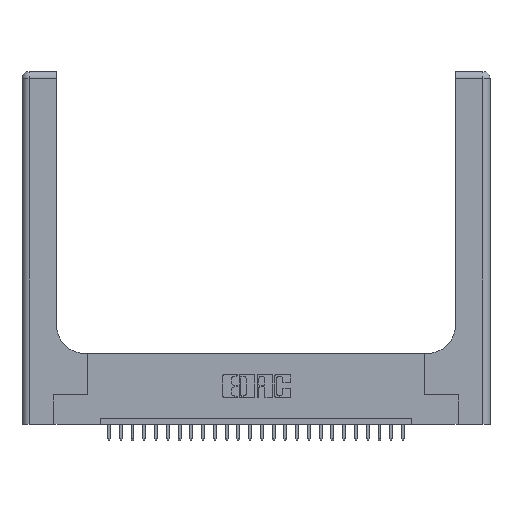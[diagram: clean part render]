
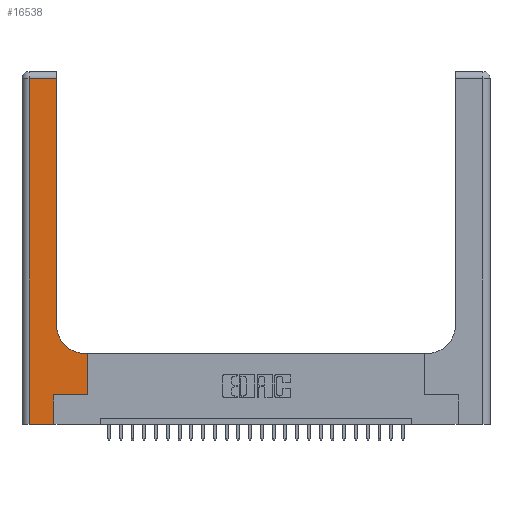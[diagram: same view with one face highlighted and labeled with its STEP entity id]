
A CAD part, top view. The second image highlights one B-rep face of the part: STEP entity #16538.
In plain terms, the highlighted planar face has unit normal (0, 0, 1).
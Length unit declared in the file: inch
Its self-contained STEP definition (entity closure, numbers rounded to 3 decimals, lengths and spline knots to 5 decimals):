
#133 = EDGE_CURVE ( 'NONE', #20920, #8429, #12386, .T. ) ;
#881 = CARTESIAN_POINT ( 'NONE',  ( 0.2915, 2.94, 0.37 ) ) ;
#912 = CARTESIAN_POINT ( 'NONE',  ( 0.269, 0.25, 0.37 ) ) ;
#1275 = CARTESIAN_POINT ( 'NONE',  ( 0.5585, 0.25, 0.37 ) ) ;
#1340 = VERTEX_POINT ( 'NONE', #8957 ) ;
#1815 = DIRECTION ( 'NONE',  ( -1., 0., 0. ) ) ;
#1842 = CARTESIAN_POINT ( 'NONE',  ( 0., 0., 0.37 ) ) ;
#2418 = CARTESIAN_POINT ( 'NONE',  ( 0.2915, 3., 0.37 ) ) ;
#2568 = AXIS2_PLACEMENT_3D ( 'NONE', #23053, #19251, #6483 ) ;
#2931 = ORIENTED_EDGE ( 'NONE', *, *, #11171, .T. ) ;
#3257 = VECTOR ( 'NONE', #15285, 39.37008 ) ;
#3536 = DIRECTION ( 'NONE',  ( 0., -1., 0. ) ) ;
#3812 = PLANE ( 'NONE',  #5685 ) ;
#4595 = CARTESIAN_POINT ( 'NONE',  ( 0.06, 3., 0.37 ) ) ;
#5685 = AXIS2_PLACEMENT_3D ( 'NONE', #11863, #24421, #1815 ) ;
#5955 = CARTESIAN_POINT ( 'NONE',  ( 0.5585, 0.25, 0.37 ) ) ;
#6483 = DIRECTION ( 'NONE',  ( 1., 0., 0. ) ) ;
#7646 = CARTESIAN_POINT ( 'NONE',  ( 0.06, 0., 0.37 ) ) ;
#7687 = EDGE_CURVE ( 'NONE', #18213, #26348, #25379, .T. ) ;
#8152 = VECTOR ( 'NONE', #20472, 39.37008 ) ;
#8415 = VERTEX_POINT ( 'NONE', #1275 ) ;
#8429 = VERTEX_POINT ( 'NONE', #22022 ) ;
#8957 = CARTESIAN_POINT ( 'NONE',  ( 0.06, 2.94, 0.37 ) ) ;
#9276 = EDGE_CURVE ( 'NONE', #23589, #14452, #10501, .T. ) ;
#9487 = LINE ( 'NONE', #1842, #12376 ) ;
#9534 = CARTESIAN_POINT ( 'NONE',  ( 0.2915, 0.85, 0.37 ) ) ;
#9589 = EDGE_CURVE ( 'NONE', #26348, #1340, #15930, .T. ) ;
#10134 = DIRECTION ( 'NONE',  ( 0., 1., 0. ) ) ;
#10501 = LINE ( 'NONE', #20712, #26354 ) ;
#11171 = EDGE_CURVE ( 'NONE', #8415, #20920, #16466, .T. ) ;
#11538 = DIRECTION ( 'NONE',  ( 1., 0., 0. ) ) ;
#11863 = CARTESIAN_POINT ( 'NONE',  ( 0., 3., 0.37 ) ) ;
#11864 = VERTEX_POINT ( 'NONE', #7646 ) ;
#12143 = VECTOR ( 'NONE', #11538, 39.37008 ) ;
#12376 = VECTOR ( 'NONE', #22918, 39.37008 ) ;
#12386 = LINE ( 'NONE', #22625, #8152 ) ;
#13251 = CARTESIAN_POINT ( 'NONE',  ( 0.5585, 0.6, 0.37 ) ) ;
#13759 = LINE ( 'NONE', #13884, #12143 ) ;
#13884 = CARTESIAN_POINT ( 'NONE',  ( 0.269, 0.25, 0.37 ) ) ;
#14039 = VECTOR ( 'NONE', #15152, 39.37008 ) ;
#14442 = ORIENTED_EDGE ( 'NONE', *, *, #133, .T. ) ;
#14452 = VERTEX_POINT ( 'NONE', #912 ) ;
#15152 = DIRECTION ( 'NONE',  ( 0., 1., 0. ) ) ;
#15285 = DIRECTION ( 'NONE',  ( -1., 0., 0. ) ) ;
#15414 = ORIENTED_EDGE ( 'NONE', *, *, #9589, .T. ) ;
#15624 = EDGE_CURVE ( 'NONE', #11864, #23589, #9487, .T. ) ;
#15787 = DIRECTION ( 'NONE',  ( 0., 1., 0. ) ) ;
#15930 = LINE ( 'NONE', #19354, #3257 ) ;
#16200 = FACE_OUTER_BOUND ( 'NONE', #22377, .T. ) ;
#16295 = VECTOR ( 'NONE', #3536, 39.37008 ) ;
#16466 = LINE ( 'NONE', #5955, #20723 ) ;
#16538 = ADVANCED_FACE ( 'NONE', ( #16200 ), #3812, .F. ) ;
#17745 = EDGE_CURVE ( 'NONE', #8429, #18213, #21360, .T. ) ;
#18213 = VERTEX_POINT ( 'NONE', #9534 ) ;
#18507 = ORIENTED_EDGE ( 'NONE', *, *, #22637, .T. ) ;
#19251 = DIRECTION ( 'NONE',  ( 0., 0., -1. ) ) ;
#19354 = CARTESIAN_POINT ( 'NONE',  ( 0., 2.94, 0.37 ) ) ;
#20167 = ORIENTED_EDGE ( 'NONE', *, *, #17745, .T. ) ;
#20472 = DIRECTION ( 'NONE',  ( -1., 0., 0. ) ) ;
#20712 = CARTESIAN_POINT ( 'NONE',  ( 0.269, 0., 0.37 ) ) ;
#20723 = VECTOR ( 'NONE', #15787, 39.37008 ) ;
#20920 = VERTEX_POINT ( 'NONE', #13251 ) ;
#21325 = CARTESIAN_POINT ( 'NONE',  ( 0.269, 0., 0.37 ) ) ;
#21360 = CIRCLE ( 'NONE', #2568, 0.25 ) ;
#21830 = LINE ( 'NONE', #4595, #16295 ) ;
#22022 = CARTESIAN_POINT ( 'NONE',  ( 0.5415, 0.6, 0.37 ) ) ;
#22159 = ORIENTED_EDGE ( 'NONE', *, *, #15624, .T. ) ;
#22222 = ORIENTED_EDGE ( 'NONE', *, *, #23088, .T. ) ;
#22377 = EDGE_LOOP ( 'NONE', ( #23172, #15414, #22222, #22159, #24361, #18507, #2931, #14442, #20167 ) ) ;
#22625 = CARTESIAN_POINT ( 'NONE',  ( 0.2915, 0.6, 0.37 ) ) ;
#22637 = EDGE_CURVE ( 'NONE', #14452, #8415, #13759, .T. ) ;
#22918 = DIRECTION ( 'NONE',  ( 1., 0., 0. ) ) ;
#23053 = CARTESIAN_POINT ( 'NONE',  ( 0.5415, 0.85, 0.37 ) ) ;
#23088 = EDGE_CURVE ( 'NONE', #1340, #11864, #21830, .T. ) ;
#23172 = ORIENTED_EDGE ( 'NONE', *, *, #7687, .T. ) ;
#23589 = VERTEX_POINT ( 'NONE', #21325 ) ;
#24361 = ORIENTED_EDGE ( 'NONE', *, *, #9276, .T. ) ;
#24421 = DIRECTION ( 'NONE',  ( 0., 0., -1. ) ) ;
#25379 = LINE ( 'NONE', #2418, #14039 ) ;
#26348 = VERTEX_POINT ( 'NONE', #881 ) ;
#26354 = VECTOR ( 'NONE', #10134, 39.37008 ) ;
